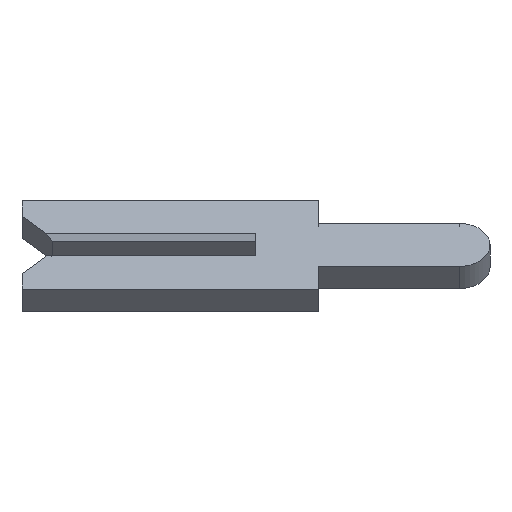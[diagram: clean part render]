
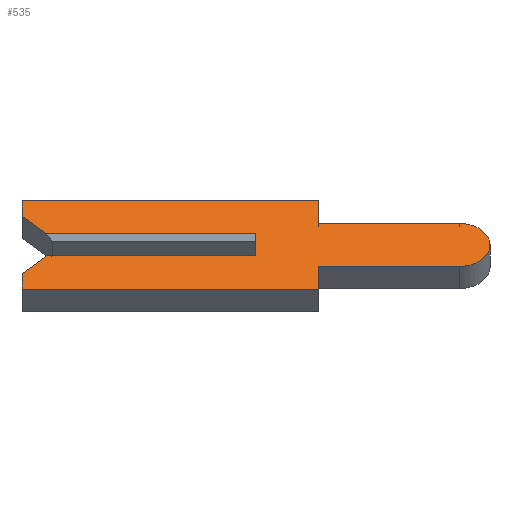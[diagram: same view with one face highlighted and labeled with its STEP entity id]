
A CAD part, left-side view. The second image highlights one B-rep face of the part: STEP entity #535.
In plain terms, the highlighted face is planar.
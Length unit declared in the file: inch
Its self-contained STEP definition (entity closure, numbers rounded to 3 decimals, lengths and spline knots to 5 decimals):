
#1 = VECTOR ( 'NONE', #39, 39.37008 ) ;
#39 = DIRECTION ( 'NONE',  ( 0., -0.707, 0.707 ) ) ;
#49 = CARTESIAN_POINT ( 'NONE',  ( -0.01, -0.1305, 0. ) ) ;
#75 = CARTESIAN_POINT ( 'NONE',  ( -0.01, -0.04, -0.0195 ) ) ;
#77 = DIRECTION ( 'NONE',  ( 0., 0., -1. ) ) ;
#81 = CARTESIAN_POINT ( 'NONE',  ( -0.01, 0., 0.0065 ) ) ;
#102 = CARTESIAN_POINT ( 'NONE',  ( -0.01, -0.04, 0.0195 ) ) ;
#113 = ORIENTED_EDGE ( 'NONE', *, *, #1038, .F. ) ;
#130 = DIRECTION ( 'NONE',  ( 0., 0., 1. ) ) ;
#133 = DIRECTION ( 'NONE',  ( 0., 0., -1. ) ) ;
#136 = VERTEX_POINT ( 'NONE', #481 ) ;
#156 = ORIENTED_EDGE ( 'NONE', *, *, #974, .F. ) ;
#158 = VECTOR ( 'NONE', #354, 39.37008 ) ;
#163 = DIRECTION ( 'NONE',  ( 1., 0., 0. ) ) ;
#169 = ORIENTED_EDGE ( 'NONE', *, *, #1017, .F. ) ;
#180 = LINE ( 'NONE', #480, #597 ) ;
#190 = DIRECTION ( 'NONE',  ( 0., 0., 1. ) ) ;
#191 = CARTESIAN_POINT ( 'NONE',  ( -0.01, 0., -0.01 ) ) ;
#193 = VERTEX_POINT ( 'NONE', #663 ) ;
#208 = VERTEX_POINT ( 'NONE', #960 ) ;
#209 = LINE ( 'NONE', #226, #1143 ) ;
#226 = CARTESIAN_POINT ( 'NONE',  ( -0.01, -0.1305, -0.01 ) ) ;
#240 = ORIENTED_EDGE ( 'NONE', *, *, #505, .F. ) ;
#255 = CARTESIAN_POINT ( 'NONE',  ( -0.01, 0.15, 0.04 ) ) ;
#266 = PLANE ( 'NONE',  #813 ) ;
#294 = EDGE_CURVE ( 'NONE', #944, #208, #627, .T. ) ;
#302 = ORIENTED_EDGE ( 'NONE', *, *, #713, .F. ) ;
#306 = DIRECTION ( 'NONE',  ( 0., -1., 0. ) ) ;
#310 = EDGE_CURVE ( 'NONE', #750, #648, #761, .T. ) ;
#344 = FACE_OUTER_BOUND ( 'NONE', #800, .T. ) ;
#354 = DIRECTION ( 'NONE',  ( 0., -1., 0. ) ) ;
#356 = LINE ( 'NONE', #450, #1096 ) ;
#358 = VECTOR ( 'NONE', #133, 39.37008 ) ;
#368 = CARTESIAN_POINT ( 'NONE',  ( -0.01, -0.1305, -0.0195 ) ) ;
#372 = CARTESIAN_POINT ( 'NONE',  ( -0.01, 0.1305, 0.0065 ) ) ;
#382 = LINE ( 'NONE', #775, #358 ) ;
#385 = VERTEX_POINT ( 'NONE', #255 ) ;
#391 = CARTESIAN_POINT ( 'NONE',  ( -0.01, 0.15, 0.01 ) ) ;
#396 = DIRECTION ( 'NONE',  ( 1., 0., 0. ) ) ;
#404 = DIRECTION ( 'NONE',  ( 0., 0., -1. ) ) ;
#409 = VECTOR ( 'NONE', #639, 39.37008 ) ;
#416 = ORIENTED_EDGE ( 'NONE', *, *, #294, .F. ) ;
#433 = CARTESIAN_POINT ( 'NONE',  ( -0.01, 0.15, 0.026 ) ) ;
#441 = EDGE_CURVE ( 'NONE', #1119, #1136, #1103, .T. ) ;
#450 = CARTESIAN_POINT ( 'NONE',  ( -0.01, 0.15, -0.026 ) ) ;
#454 = VECTOR ( 'NONE', #853, 39.37008 ) ;
#459 = ORIENTED_EDGE ( 'NONE', *, *, #1078, .F. ) ;
#478 = CARTESIAN_POINT ( 'NONE',  ( -0.01, -0.04, -0.04 ) ) ;
#480 = CARTESIAN_POINT ( 'NONE',  ( -0.01, 0.15, 0.026 ) ) ;
#481 = CARTESIAN_POINT ( 'NONE',  ( -0.01, -0.1305, 0.0195 ) ) ;
#505 = EDGE_CURVE ( 'NONE', #677, #193, #654, .T. ) ;
#511 = VECTOR ( 'NONE', #869, 39.37008 ) ;
#515 = ORIENTED_EDGE ( 'NONE', *, *, #624, .F. ) ;
#517 = DIRECTION ( 'NONE',  ( 0., 0., -1. ) ) ;
#519 = CARTESIAN_POINT ( 'NONE',  ( -0.01, 0., 0.01 ) ) ;
#535 = ADVANCED_FACE ( 'NONE', ( #344 ), #266, .F. ) ;
#536 = ORIENTED_EDGE ( 'NONE', *, *, #310, .T. ) ;
#560 = VERTEX_POINT ( 'NONE', #433 ) ;
#579 = CARTESIAN_POINT ( 'NONE',  ( -0.01, 0.15, -0.04 ) ) ;
#597 = VECTOR ( 'NONE', #130, 39.37008 ) ;
#624 = EDGE_CURVE ( 'NONE', #768, #648, #975, .T. ) ;
#627 = LINE ( 'NONE', #955, #1 ) ;
#635 = CARTESIAN_POINT ( 'NONE',  ( -0.01, 0.134, 0.01 ) ) ;
#639 = DIRECTION ( 'NONE',  ( 0., -1., 0. ) ) ;
#640 = VECTOR ( 'NONE', #973, 39.37008 ) ;
#648 = VERTEX_POINT ( 'NONE', #519 ) ;
#654 = LINE ( 'NONE', #75, #640 ) ;
#663 = CARTESIAN_POINT ( 'NONE',  ( -0.01, -0.04, -0.0195 ) ) ;
#674 = EDGE_CURVE ( 'NONE', #751, #944, #356, .T. ) ;
#677 = VERTEX_POINT ( 'NONE', #368 ) ;
#687 = LINE ( 'NONE', #1001, #158 ) ;
#707 = DIRECTION ( 'NONE',  ( 0., 0., 1. ) ) ;
#713 = EDGE_CURVE ( 'NONE', #1136, #136, #738, .T. ) ;
#721 = CARTESIAN_POINT ( 'NONE',  ( -0.01, 0.15, -0.04 ) ) ;
#738 = LINE ( 'NONE', #102, #409 ) ;
#750 = VERTEX_POINT ( 'NONE', #635 ) ;
#751 = VERTEX_POINT ( 'NONE', #721 ) ;
#761 = LINE ( 'NONE', #391, #511 ) ;
#768 = VERTEX_POINT ( 'NONE', #191 ) ;
#774 = AXIS2_PLACEMENT_3D ( 'NONE', #49, #396, #404 ) ;
#775 = CARTESIAN_POINT ( 'NONE',  ( -0.01, -0.04, -0.04 ) ) ;
#800 = EDGE_LOOP ( 'NONE', ( #536, #515, #169, #416, #859, #892, #459, #240, #914, #302, #1074, #1062, #113, #156 ) ) ;
#805 = EDGE_CURVE ( 'NONE', #385, #1119, #687, .T. ) ;
#813 = AXIS2_PLACEMENT_3D ( 'NONE', #972, #163, #77 ) ;
#853 = DIRECTION ( 'NONE',  ( 0., 0.707, 0.707 ) ) ;
#859 = ORIENTED_EDGE ( 'NONE', *, *, #674, .F. ) ;
#869 = DIRECTION ( 'NONE',  ( 0., -1., 0. ) ) ;
#873 = CARTESIAN_POINT ( 'NONE',  ( -0.01, -0.04, 0.04 ) ) ;
#888 = VECTOR ( 'NONE', #1133, 39.37008 ) ;
#892 = ORIENTED_EDGE ( 'NONE', *, *, #1020, .F. ) ;
#907 = LINE ( 'NONE', #372, #454 ) ;
#914 = ORIENTED_EDGE ( 'NONE', *, *, #989, .F. ) ;
#920 = LINE ( 'NONE', #579, #888 ) ;
#943 = CARTESIAN_POINT ( 'NONE',  ( -0.01, -0.04, 0.0195 ) ) ;
#944 = VERTEX_POINT ( 'NONE', #1008 ) ;
#948 = CIRCLE ( 'NONE', #774, 0.0195 ) ;
#950 = VECTOR ( 'NONE', #517, 39.37008 ) ;
#955 = CARTESIAN_POINT ( 'NONE',  ( -0.01, 0.1305, -0.0065 ) ) ;
#960 = CARTESIAN_POINT ( 'NONE',  ( -0.01, 0.134, -0.01 ) ) ;
#972 = CARTESIAN_POINT ( 'NONE',  ( -0.01, -0.1305, 0. ) ) ;
#973 = DIRECTION ( 'NONE',  ( 0., 1., 0. ) ) ;
#974 = EDGE_CURVE ( 'NONE', #750, #560, #907, .T. ) ;
#975 = LINE ( 'NONE', #81, #990 ) ;
#989 = EDGE_CURVE ( 'NONE', #136, #677, #948, .T. ) ;
#990 = VECTOR ( 'NONE', #707, 39.37008 ) ;
#1001 = CARTESIAN_POINT ( 'NONE',  ( -0.01, 0.15, 0.04 ) ) ;
#1008 = CARTESIAN_POINT ( 'NONE',  ( -0.01, 0.15, -0.026 ) ) ;
#1017 = EDGE_CURVE ( 'NONE', #208, #768, #209, .T. ) ;
#1020 = EDGE_CURVE ( 'NONE', #1023, #751, #920, .T. ) ;
#1023 = VERTEX_POINT ( 'NONE', #478 ) ;
#1038 = EDGE_CURVE ( 'NONE', #560, #385, #180, .T. ) ;
#1062 = ORIENTED_EDGE ( 'NONE', *, *, #805, .F. ) ;
#1074 = ORIENTED_EDGE ( 'NONE', *, *, #441, .F. ) ;
#1078 = EDGE_CURVE ( 'NONE', #193, #1023, #382, .T. ) ;
#1096 = VECTOR ( 'NONE', #190, 39.37008 ) ;
#1103 = LINE ( 'NONE', #873, #950 ) ;
#1119 = VERTEX_POINT ( 'NONE', #1138 ) ;
#1133 = DIRECTION ( 'NONE',  ( 0., 1., 0. ) ) ;
#1136 = VERTEX_POINT ( 'NONE', #943 ) ;
#1138 = CARTESIAN_POINT ( 'NONE',  ( -0.01, -0.04, 0.04 ) ) ;
#1143 = VECTOR ( 'NONE', #306, 39.37008 ) ;
